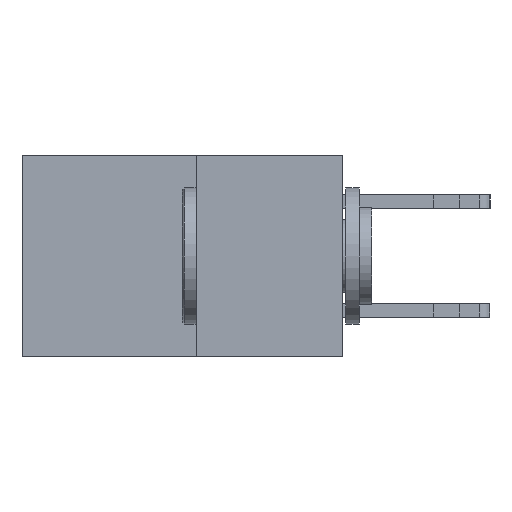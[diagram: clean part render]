
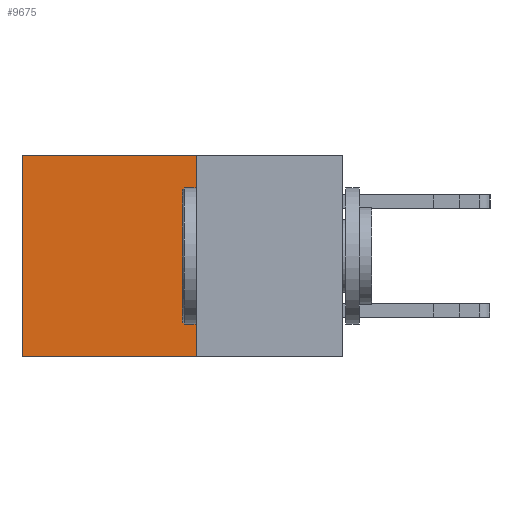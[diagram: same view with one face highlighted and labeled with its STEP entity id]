
A CAD part, left-side view. The second image highlights one B-rep face of the part: STEP entity #9675.
In plain terms, the highlighted planar face has unit normal (-1, 0, 0).
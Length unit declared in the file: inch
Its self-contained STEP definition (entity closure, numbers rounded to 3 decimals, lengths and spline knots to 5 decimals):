
#437 = VERTEX_POINT ( 'NONE', #10359 ) ;
#1002 = CARTESIAN_POINT ( 'NONE',  ( 0.277, 0.27, -0.37 ) ) ;
#1184 = PLANE ( 'NONE',  #15335 ) ;
#1770 = EDGE_CURVE ( 'NONE', #4861, #437, #9010, .T. ) ;
#2163 = EDGE_LOOP ( 'NONE', ( #11716, #4512, #7037, #2796 ) ) ;
#2645 = VERTEX_POINT ( 'NONE', #7536 ) ;
#2796 = ORIENTED_EDGE ( 'NONE', *, *, #13283, .T. ) ;
#3469 = DIRECTION ( 'NONE',  ( 0., 1., 0. ) ) ;
#3515 = VERTEX_POINT ( 'NONE', #6564 ) ;
#4424 = CARTESIAN_POINT ( 'NONE',  ( 0.277, 0.27, -0.37 ) ) ;
#4477 = DIRECTION ( 'NONE',  ( 0., 0., -1. ) ) ;
#4512 = ORIENTED_EDGE ( 'NONE', *, *, #12209, .F. ) ;
#4752 = CARTESIAN_POINT ( 'NONE',  ( 0.277, 0.59, 0. ) ) ;
#4861 = VERTEX_POINT ( 'NONE', #4752 ) ;
#4863 = DIRECTION ( 'NONE',  ( 1., 0., 0. ) ) ;
#5184 = LINE ( 'NONE', #1002, #11292 ) ;
#5556 = VECTOR ( 'NONE', #4477, 39.37008 ) ;
#5850 = CARTESIAN_POINT ( 'NONE',  ( 0.277, 0.27, 0. ) ) ;
#6106 = VECTOR ( 'NONE', #3469, 39.37008 ) ;
#6564 = CARTESIAN_POINT ( 'NONE',  ( 0.277, 0.27, 0. ) ) ;
#6614 = FACE_OUTER_BOUND ( 'NONE', #2163, .T. ) ;
#7037 = ORIENTED_EDGE ( 'NONE', *, *, #12601, .F. ) ;
#7536 = CARTESIAN_POINT ( 'NONE',  ( 0.277, 0.27, -0.37 ) ) ;
#9010 = LINE ( 'NONE', #14015, #11434 ) ;
#9675 = ADVANCED_FACE ( 'NONE', ( #6614 ), #1184, .F. ) ;
#10359 = CARTESIAN_POINT ( 'NONE',  ( 0.277, 0.59, -0.37 ) ) ;
#11292 = VECTOR ( 'NONE', #14272, 39.37008 ) ;
#11434 = VECTOR ( 'NONE', #15140, 39.37008 ) ;
#11716 = ORIENTED_EDGE ( 'NONE', *, *, #1770, .T. ) ;
#12146 = CARTESIAN_POINT ( 'NONE',  ( 0.277, 0.27, -0.37 ) ) ;
#12209 = EDGE_CURVE ( 'NONE', #2645, #437, #5184, .T. ) ;
#12391 = LINE ( 'NONE', #4424, #5556 ) ;
#12601 = EDGE_CURVE ( 'NONE', #3515, #2645, #12391, .T. ) ;
#12925 = LINE ( 'NONE', #5850, #6106 ) ;
#13283 = EDGE_CURVE ( 'NONE', #3515, #4861, #12925, .T. ) ;
#13353 = DIRECTION ( 'NONE',  ( 0., 0., -1. ) ) ;
#14015 = CARTESIAN_POINT ( 'NONE',  ( 0.277, 0.59, -0.37 ) ) ;
#14272 = DIRECTION ( 'NONE',  ( 0., 1., 0. ) ) ;
#15140 = DIRECTION ( 'NONE',  ( 0., 0., -1. ) ) ;
#15335 = AXIS2_PLACEMENT_3D ( 'NONE', #12146, #4863, #13353 ) ;
